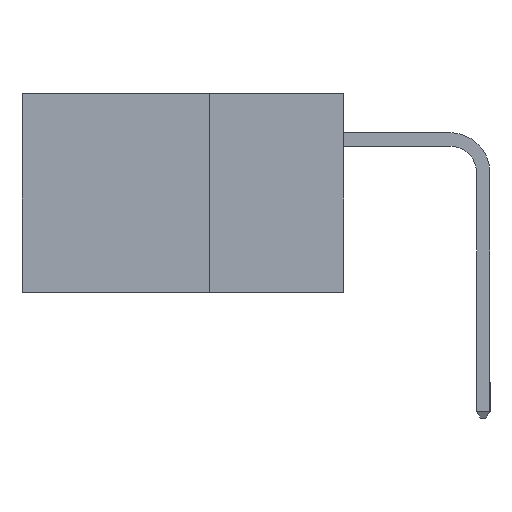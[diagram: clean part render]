
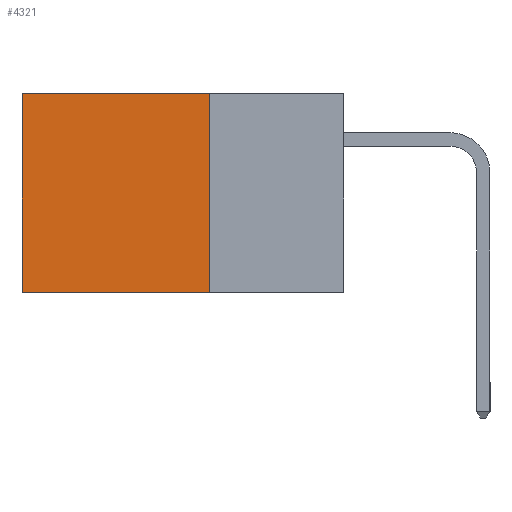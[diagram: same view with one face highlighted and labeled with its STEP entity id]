
A CAD part, left-side view. The second image highlights one B-rep face of the part: STEP entity #4321.
In plain terms, the highlighted planar face has unit normal (-1, 0, 0).
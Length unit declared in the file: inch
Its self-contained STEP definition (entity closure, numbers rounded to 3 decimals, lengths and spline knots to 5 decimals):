
#930 = VECTOR ( 'NONE', #22262, 39.37008 ) ;
#1141 = EDGE_LOOP ( 'NONE', ( #21115, #22293, #19149, #10310 ) ) ;
#1929 = VECTOR ( 'NONE', #21131, 39.37008 ) ;
#3649 = VERTEX_POINT ( 'NONE', #4907 ) ;
#4321 = ADVANCED_FACE ( 'NONE', ( #16883 ), #9564, .F. ) ;
#4907 = CARTESIAN_POINT ( 'NONE',  ( 0.298, 0.6, -0.37 ) ) ;
#6781 = DIRECTION ( 'NONE',  ( 1., 0., 0. ) ) ;
#7019 = VERTEX_POINT ( 'NONE', #13823 ) ;
#8116 = VERTEX_POINT ( 'NONE', #8230 ) ;
#8129 = DIRECTION ( 'NONE',  ( 0., 1., 0. ) ) ;
#8230 = CARTESIAN_POINT ( 'NONE',  ( 0.298, 0.25, 0. ) ) ;
#8615 = CARTESIAN_POINT ( 'NONE',  ( 0.298, 0.25, -0.37 ) ) ;
#8933 = AXIS2_PLACEMENT_3D ( 'NONE', #9361, #6781, #10275 ) ;
#9361 = CARTESIAN_POINT ( 'NONE',  ( 0.298, 0.25, 0. ) ) ;
#9564 = PLANE ( 'NONE',  #8933 ) ;
#9689 = DIRECTION ( 'NONE',  ( 0., 0., -1. ) ) ;
#9935 = CARTESIAN_POINT ( 'NONE',  ( 0.298, 0.6, 0. ) ) ;
#10155 = VERTEX_POINT ( 'NONE', #19013 ) ;
#10275 = DIRECTION ( 'NONE',  ( 0., 0., -1. ) ) ;
#10310 = ORIENTED_EDGE ( 'NONE', *, *, #13415, .T. ) ;
#10455 = VECTOR ( 'NONE', #9689, 39.37008 ) ;
#11090 = EDGE_CURVE ( 'NONE', #7019, #3649, #14462, .T. ) ;
#11526 = LINE ( 'NONE', #18872, #930 ) ;
#13415 = EDGE_CURVE ( 'NONE', #8116, #10155, #22302, .T. ) ;
#13823 = CARTESIAN_POINT ( 'NONE',  ( 0.298, 0.25, -0.37 ) ) ;
#14462 = LINE ( 'NONE', #8615, #18145 ) ;
#16883 = FACE_OUTER_BOUND ( 'NONE', #1141, .T. ) ;
#18145 = VECTOR ( 'NONE', #8129, 39.37008 ) ;
#18872 = CARTESIAN_POINT ( 'NONE',  ( 0.298, 0.25, 0. ) ) ;
#19013 = CARTESIAN_POINT ( 'NONE',  ( 0.298, 0.6, 0. ) ) ;
#19059 = EDGE_CURVE ( 'NONE', #10155, #3649, #20437, .T. ) ;
#19149 = ORIENTED_EDGE ( 'NONE', *, *, #23741, .F. ) ;
#20437 = LINE ( 'NONE', #9935, #10455 ) ;
#20982 = CARTESIAN_POINT ( 'NONE',  ( 0.298, 0.25, 0. ) ) ;
#21115 = ORIENTED_EDGE ( 'NONE', *, *, #19059, .T. ) ;
#21131 = DIRECTION ( 'NONE',  ( 0., 1., 0. ) ) ;
#22262 = DIRECTION ( 'NONE',  ( 0., 0., -1. ) ) ;
#22293 = ORIENTED_EDGE ( 'NONE', *, *, #11090, .F. ) ;
#22302 = LINE ( 'NONE', #20982, #1929 ) ;
#23741 = EDGE_CURVE ( 'NONE', #8116, #7019, #11526, .T. ) ;
